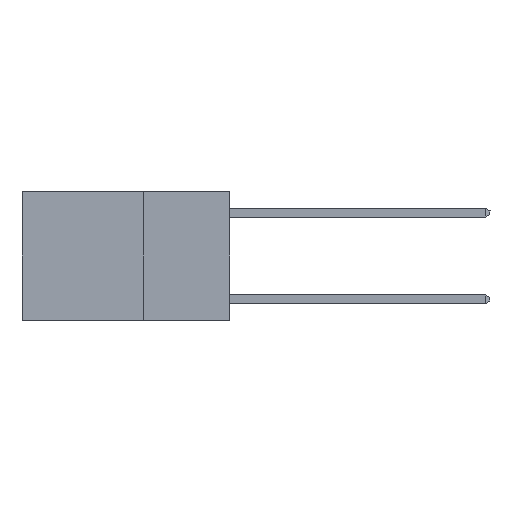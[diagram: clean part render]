
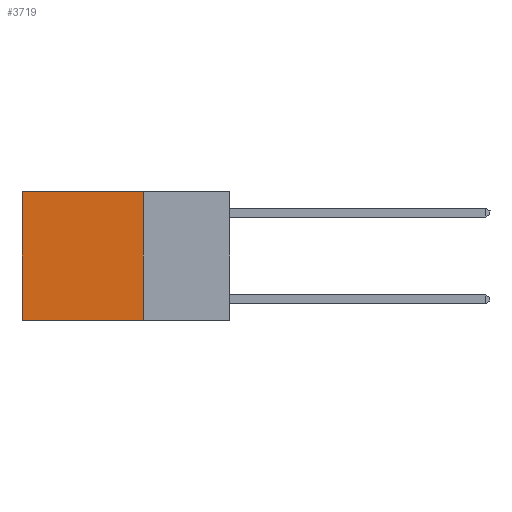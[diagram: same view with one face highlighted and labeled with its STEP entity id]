
A CAD part, left-side view. The second image highlights one B-rep face of the part: STEP entity #3719.
In plain terms, the highlighted planar face has unit normal (-1, 0, 0).
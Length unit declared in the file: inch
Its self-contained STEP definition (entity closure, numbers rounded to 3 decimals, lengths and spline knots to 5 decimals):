
#864 = CARTESIAN_POINT ( 'NONE',  ( 0.2625, 0.25, 0. ) ) ;
#931 = AXIS2_PLACEMENT_3D ( 'NONE', #864, #17238, #15294 ) ;
#2124 = ORIENTED_EDGE ( 'NONE', *, *, #2862, .F. ) ;
#2862 = EDGE_CURVE ( 'NONE', #20140, #13941, #7522, .T. ) ;
#3719 = ADVANCED_FACE ( 'NONE', ( #5698 ), #13063, .F. ) ;
#4040 = DIRECTION ( 'NONE',  ( 0., 1., 0. ) ) ;
#5698 = FACE_OUTER_BOUND ( 'NONE', #13689, .T. ) ;
#6086 = VERTEX_POINT ( 'NONE', #23647 ) ;
#6174 = EDGE_CURVE ( 'NONE', #10285, #13941, #14671, .T. ) ;
#6209 = EDGE_CURVE ( 'NONE', #6086, #10285, #12756, .T. ) ;
#7055 = ORIENTED_EDGE ( 'NONE', *, *, #19408, .F. ) ;
#7522 = LINE ( 'NONE', #20507, #21022 ) ;
#8612 = VECTOR ( 'NONE', #17987, 39.37008 ) ;
#9189 = CARTESIAN_POINT ( 'NONE',  ( 0.2625, 0.6, 0. ) ) ;
#9236 = CARTESIAN_POINT ( 'NONE',  ( 0.2625, 0.6, -0.37 ) ) ;
#10285 = VERTEX_POINT ( 'NONE', #9189 ) ;
#10507 = DIRECTION ( 'NONE',  ( 0., 1., 0. ) ) ;
#11204 = CARTESIAN_POINT ( 'NONE',  ( 0.2625, 0.25, 0. ) ) ;
#12756 = LINE ( 'NONE', #22031, #13400 ) ;
#13063 = PLANE ( 'NONE',  #931 ) ;
#13400 = VECTOR ( 'NONE', #4040, 39.37008 ) ;
#13689 = EDGE_LOOP ( 'NONE', ( #13888, #2124, #7055, #15576 ) ) ;
#13888 = ORIENTED_EDGE ( 'NONE', *, *, #6174, .T. ) ;
#13941 = VERTEX_POINT ( 'NONE', #9236 ) ;
#14671 = LINE ( 'NONE', #22114, #8612 ) ;
#14718 = VECTOR ( 'NONE', #21044, 39.37008 ) ;
#15294 = DIRECTION ( 'NONE',  ( 0., 0., -1. ) ) ;
#15576 = ORIENTED_EDGE ( 'NONE', *, *, #6209, .T. ) ;
#17238 = DIRECTION ( 'NONE',  ( 1., 0., 0. ) ) ;
#17987 = DIRECTION ( 'NONE',  ( 0., 0., -1. ) ) ;
#19408 = EDGE_CURVE ( 'NONE', #6086, #20140, #23669, .T. ) ;
#20140 = VERTEX_POINT ( 'NONE', #21362 ) ;
#20507 = CARTESIAN_POINT ( 'NONE',  ( 0.2625, 0.25, -0.37 ) ) ;
#21022 = VECTOR ( 'NONE', #10507, 39.37008 ) ;
#21044 = DIRECTION ( 'NONE',  ( 0., 0., -1. ) ) ;
#21362 = CARTESIAN_POINT ( 'NONE',  ( 0.2625, 0.25, -0.37 ) ) ;
#22031 = CARTESIAN_POINT ( 'NONE',  ( 0.2625, 0.25, 0. ) ) ;
#22114 = CARTESIAN_POINT ( 'NONE',  ( 0.2625, 0.6, 0. ) ) ;
#23647 = CARTESIAN_POINT ( 'NONE',  ( 0.2625, 0.25, 0. ) ) ;
#23669 = LINE ( 'NONE', #11204, #14718 ) ;
